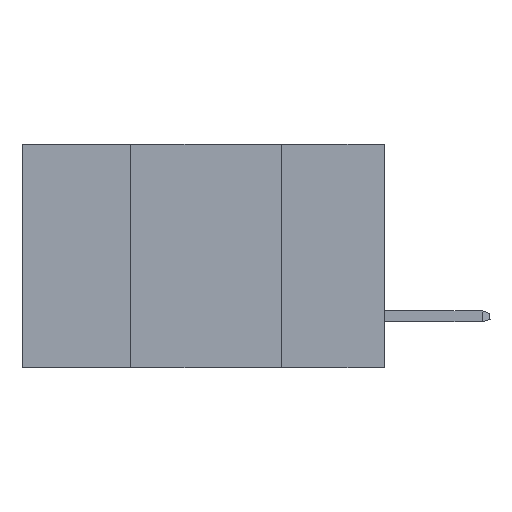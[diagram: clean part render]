
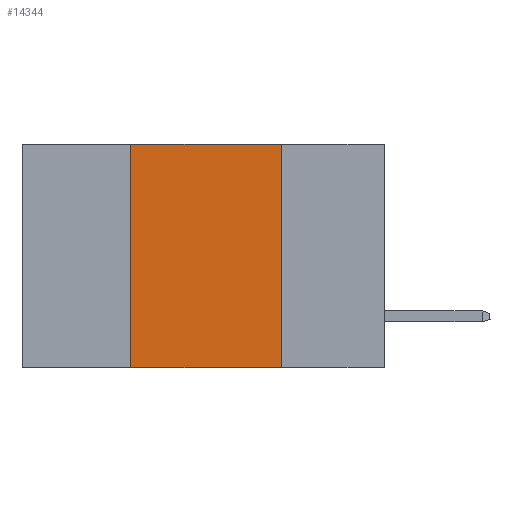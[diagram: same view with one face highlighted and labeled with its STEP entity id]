
A CAD part, left-side view. The second image highlights one B-rep face of the part: STEP entity #14344.
In plain terms, the highlighted planar face has unit normal (-1, 0, 0).
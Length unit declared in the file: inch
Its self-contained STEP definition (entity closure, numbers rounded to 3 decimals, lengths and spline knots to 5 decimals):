
#1519 = CARTESIAN_POINT ( 'NONE',  ( 0., 0.42, -0.37 ) ) ;
#2073 = EDGE_LOOP ( 'NONE', ( #17558, #7242, #2253, #33168 ) ) ;
#2253 = ORIENTED_EDGE ( 'NONE', *, *, #7247, .F. ) ;
#2299 = AXIS2_PLACEMENT_3D ( 'NONE', #24109, #3457, #3347 ) ;
#3049 = VECTOR ( 'NONE', #27041, 39.37008 ) ;
#3347 = DIRECTION ( 'NONE',  ( 0., 0., -1. ) ) ;
#3457 = DIRECTION ( 'NONE',  ( 1., 0., 0. ) ) ;
#4450 = CARTESIAN_POINT ( 'NONE',  ( 0., 0.42, 0. ) ) ;
#7242 = ORIENTED_EDGE ( 'NONE', *, *, #20076, .F. ) ;
#7247 = EDGE_CURVE ( 'NONE', #16801, #32425, #28344, .T. ) ;
#8898 = PLANE ( 'NONE',  #2299 ) ;
#9205 = VECTOR ( 'NONE', #17378, 39.37008 ) ;
#10084 = CARTESIAN_POINT ( 'NONE',  ( 0., 0.17, 0. ) ) ;
#11530 = CARTESIAN_POINT ( 'NONE',  ( 0., 0.17, 0. ) ) ;
#12894 = CARTESIAN_POINT ( 'NONE',  ( 0., 0.6, 0. ) ) ;
#13100 = EDGE_CURVE ( 'NONE', #32829, #30825, #14839, .T. ) ;
#14344 = ADVANCED_FACE ( 'NONE', ( #20336 ), #8898, .F. ) ;
#14839 = LINE ( 'NONE', #11530, #26119 ) ;
#16088 = LINE ( 'NONE', #32824, #9205 ) ;
#16325 = DIRECTION ( 'NONE',  ( 0., 0., -1. ) ) ;
#16801 = VERTEX_POINT ( 'NONE', #1519 ) ;
#17378 = DIRECTION ( 'NONE',  ( 0., -1., 0. ) ) ;
#17558 = ORIENTED_EDGE ( 'NONE', *, *, #13100, .F. ) ;
#17973 = DIRECTION ( 'NONE',  ( 0., -1., 0. ) ) ;
#18387 = EDGE_CURVE ( 'NONE', #16801, #30825, #16088, .T. ) ;
#18920 = CARTESIAN_POINT ( 'NONE',  ( 0., 0.17, -0.37 ) ) ;
#20076 = EDGE_CURVE ( 'NONE', #32425, #32829, #25137, .T. ) ;
#20336 = FACE_OUTER_BOUND ( 'NONE', #2073, .T. ) ;
#24109 = CARTESIAN_POINT ( 'NONE',  ( 0., 0.6, 0. ) ) ;
#25137 = LINE ( 'NONE', #12894, #27155 ) ;
#26119 = VECTOR ( 'NONE', #16325, 39.37008 ) ;
#27041 = DIRECTION ( 'NONE',  ( 0., 0., 1. ) ) ;
#27155 = VECTOR ( 'NONE', #17973, 39.37008 ) ;
#28344 = LINE ( 'NONE', #32008, #3049 ) ;
#30825 = VERTEX_POINT ( 'NONE', #18920 ) ;
#32008 = CARTESIAN_POINT ( 'NONE',  ( 0., 0.42, 0. ) ) ;
#32425 = VERTEX_POINT ( 'NONE', #4450 ) ;
#32824 = CARTESIAN_POINT ( 'NONE',  ( 0., 0.6, -0.37 ) ) ;
#32829 = VERTEX_POINT ( 'NONE', #10084 ) ;
#33168 = ORIENTED_EDGE ( 'NONE', *, *, #18387, .T. ) ;
